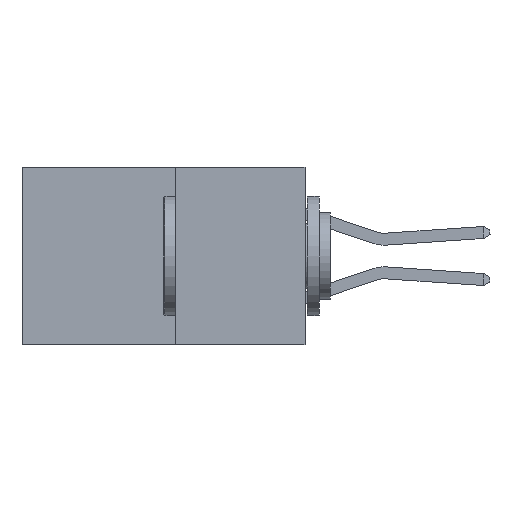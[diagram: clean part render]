
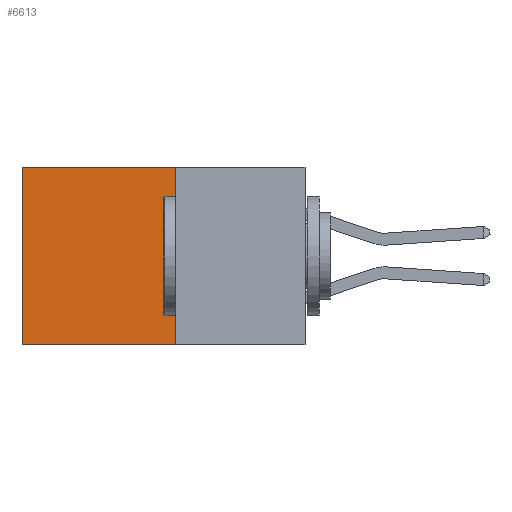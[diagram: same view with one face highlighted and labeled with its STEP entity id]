
A CAD part, left-side view. The second image highlights one B-rep face of the part: STEP entity #6613.
In plain terms, the highlighted planar face has unit normal (-1, 0, 0).
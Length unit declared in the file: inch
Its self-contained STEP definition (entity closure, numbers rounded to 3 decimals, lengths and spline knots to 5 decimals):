
#1109 = DIRECTION ( 'NONE',  ( 0., 1., 0. ) ) ;
#1155 = CARTESIAN_POINT ( 'NONE',  ( 0.277, 0.27, 0. ) ) ;
#1335 = ORIENTED_EDGE ( 'NONE', *, *, #13225, .T. ) ;
#1697 = CARTESIAN_POINT ( 'NONE',  ( 0.277, 0.27, 0. ) ) ;
#1840 = ORIENTED_EDGE ( 'NONE', *, *, #20178, .F. ) ;
#2542 = VECTOR ( 'NONE', #1109, 39.37008 ) ;
#2835 = FACE_OUTER_BOUND ( 'NONE', #3085, .T. ) ;
#3085 = EDGE_LOOP ( 'NONE', ( #1335, #18768, #1840, #12261 ) ) ;
#4586 = DIRECTION ( 'NONE',  ( 0., 0., -1. ) ) ;
#5187 = VECTOR ( 'NONE', #4586, 39.37008 ) ;
#6278 = CARTESIAN_POINT ( 'NONE',  ( 0.277, 0.27, -0.37 ) ) ;
#6537 = CARTESIAN_POINT ( 'NONE',  ( 0.277, 0.59, 0. ) ) ;
#6613 = ADVANCED_FACE ( 'NONE', ( #2835 ), #10640, .F. ) ;
#6797 = LINE ( 'NONE', #14346, #10704 ) ;
#7331 = VERTEX_POINT ( 'NONE', #1697 ) ;
#7403 = EDGE_CURVE ( 'NONE', #7331, #16691, #19894, .T. ) ;
#7776 = VERTEX_POINT ( 'NONE', #17839 ) ;
#7861 = DIRECTION ( 'NONE',  ( 0., 1., 0. ) ) ;
#9636 = LINE ( 'NONE', #11245, #5187 ) ;
#10567 = DIRECTION ( 'NONE',  ( 0., 0., -1. ) ) ;
#10596 = DIRECTION ( 'NONE',  ( 1., 0., 0. ) ) ;
#10640 = PLANE ( 'NONE',  #13431 ) ;
#10704 = VECTOR ( 'NONE', #7861, 39.37008 ) ;
#10737 = CARTESIAN_POINT ( 'NONE',  ( 0.277, 0.27, -0.37 ) ) ;
#11245 = CARTESIAN_POINT ( 'NONE',  ( 0.277, 0.59, -0.37 ) ) ;
#12261 = ORIENTED_EDGE ( 'NONE', *, *, #7403, .T. ) ;
#12766 = CARTESIAN_POINT ( 'NONE',  ( 0.277, 0.27, -0.37 ) ) ;
#13225 = EDGE_CURVE ( 'NONE', #16691, #7776, #9636, .T. ) ;
#13431 = AXIS2_PLACEMENT_3D ( 'NONE', #10737, #10596, #10567 ) ;
#14346 = CARTESIAN_POINT ( 'NONE',  ( 0.277, 0.27, -0.37 ) ) ;
#16691 = VERTEX_POINT ( 'NONE', #6537 ) ;
#16795 = VECTOR ( 'NONE', #17588, 39.37008 ) ;
#17588 = DIRECTION ( 'NONE',  ( 0., 0., -1. ) ) ;
#17839 = CARTESIAN_POINT ( 'NONE',  ( 0.277, 0.59, -0.37 ) ) ;
#18768 = ORIENTED_EDGE ( 'NONE', *, *, #19020, .F. ) ;
#19020 = EDGE_CURVE ( 'NONE', #19063, #7776, #6797, .T. ) ;
#19063 = VERTEX_POINT ( 'NONE', #6278 ) ;
#19894 = LINE ( 'NONE', #1155, #2542 ) ;
#20178 = EDGE_CURVE ( 'NONE', #7331, #19063, #20900, .T. ) ;
#20900 = LINE ( 'NONE', #12766, #16795 ) ;
